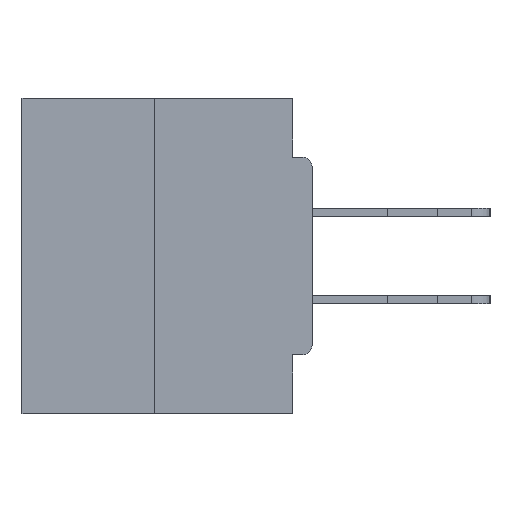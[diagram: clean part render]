
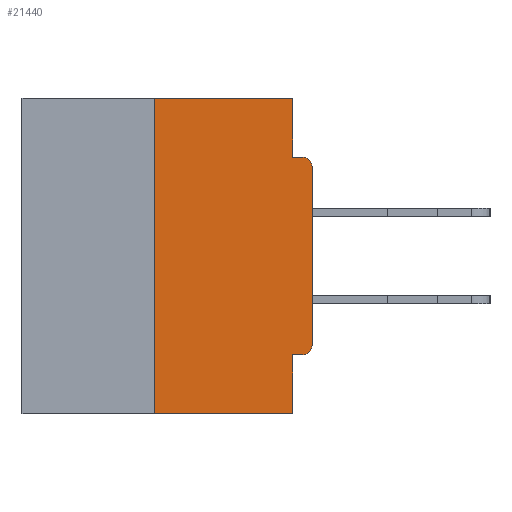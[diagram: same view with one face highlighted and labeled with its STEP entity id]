
A CAD part, left-side view. The second image highlights one B-rep face of the part: STEP entity #21440.
In plain terms, the highlighted planar face has unit normal (-1, 0, 0).
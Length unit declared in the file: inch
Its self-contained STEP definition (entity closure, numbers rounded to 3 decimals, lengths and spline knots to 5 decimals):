
#473 = VERTEX_POINT ( 'NONE', #34728 ) ;
#494 = CARTESIAN_POINT ( 'NONE',  ( 0., 0.25, 0. ) ) ;
#676 = DIRECTION ( 'NONE',  ( 0., 1., 0. ) ) ;
#697 = DIRECTION ( 'NONE',  ( 0., -1., 0. ) ) ;
#2368 = LINE ( 'NONE', #22372, #6862 ) ;
#2911 = LINE ( 'NONE', #5901, #22941 ) ;
#3877 = CARTESIAN_POINT ( 'NONE',  ( 0., 0., -0.4065 ) ) ;
#5074 = CARTESIAN_POINT ( 'NONE',  ( 0., 0.46, 0. ) ) ;
#5537 = CARTESIAN_POINT ( 'NONE',  ( 0., 0.015, -0.4065 ) ) ;
#5901 = CARTESIAN_POINT ( 'NONE',  ( 0., 0.25, 0. ) ) ;
#6268 = CIRCLE ( 'NONE', #41624, 0.015 ) ;
#6456 = VERTEX_POINT ( 'NONE', #11626 ) ;
#6700 = EDGE_CURVE ( 'NONE', #13924, #473, #20686, .T. ) ;
#6862 = VECTOR ( 'NONE', #24736, 39.37008 ) ;
#7911 = VERTEX_POINT ( 'NONE', #41515 ) ;
#8162 = VECTOR ( 'NONE', #697, 39.37008 ) ;
#8519 = CARTESIAN_POINT ( 'NONE',  ( 0., 0.031, -0.5 ) ) ;
#8876 = DIRECTION ( 'NONE',  ( -1., 0., 0. ) ) ;
#9008 = CARTESIAN_POINT ( 'NONE',  ( 0., 0.031, -0.5 ) ) ;
#9413 = ORIENTED_EDGE ( 'NONE', *, *, #31397, .F. ) ;
#9829 = LINE ( 'NONE', #17039, #32556 ) ;
#10987 = DIRECTION ( 'NONE',  ( -1., 0., 0. ) ) ;
#11491 = ORIENTED_EDGE ( 'NONE', *, *, #18072, .T. ) ;
#11492 = VERTEX_POINT ( 'NONE', #39546 ) ;
#11626 = CARTESIAN_POINT ( 'NONE',  ( 0., 0.031, 0. ) ) ;
#11719 = VECTOR ( 'NONE', #18060, 39.37008 ) ;
#12314 = VECTOR ( 'NONE', #35559, 39.37008 ) ;
#13902 = CARTESIAN_POINT ( 'NONE',  ( 0., 0., -0.1085 ) ) ;
#13924 = VERTEX_POINT ( 'NONE', #5537 ) ;
#14106 = LINE ( 'NONE', #29868, #8162 ) ;
#14515 = VERTEX_POINT ( 'NONE', #494 ) ;
#15342 = LINE ( 'NONE', #41324, #12314 ) ;
#15355 = ORIENTED_EDGE ( 'NONE', *, *, #36718, .T. ) ;
#15449 = EDGE_CURVE ( 'NONE', #14515, #6456, #34242, .T. ) ;
#15707 = VECTOR ( 'NONE', #676, 39.37008 ) ;
#16113 = CARTESIAN_POINT ( 'NONE',  ( 0., 0., -0.3915 ) ) ;
#16138 = ORIENTED_EDGE ( 'NONE', *, *, #15449, .F. ) ;
#17039 = CARTESIAN_POINT ( 'NONE',  ( 0., 0.031, 0. ) ) ;
#17478 = ORIENTED_EDGE ( 'NONE', *, *, #41004, .F. ) ;
#18060 = DIRECTION ( 'NONE',  ( 0., -1., 0. ) ) ;
#18072 = EDGE_CURVE ( 'NONE', #13924, #34018, #26867, .T. ) ;
#19456 = DIRECTION ( 'NONE',  ( 1., 0., 0. ) ) ;
#20686 = LINE ( 'NONE', #3877, #15707 ) ;
#20988 = CARTESIAN_POINT ( 'NONE',  ( 0., 0.015, -0.3915 ) ) ;
#21440 = ADVANCED_FACE ( 'NONE', ( #38626 ), #32837, .F. ) ;
#21739 = AXIS2_PLACEMENT_3D ( 'NONE', #25638, #19456, #25832 ) ;
#21856 = DIRECTION ( 'NONE',  ( 0., 0., -1. ) ) ;
#22372 = CARTESIAN_POINT ( 'NONE',  ( 0., 0.46, -0.5 ) ) ;
#22941 = VECTOR ( 'NONE', #41046, 39.37008 ) ;
#23194 = EDGE_CURVE ( 'NONE', #11492, #26535, #2368, .T. ) ;
#24131 = AXIS2_PLACEMENT_3D ( 'NONE', #20988, #10987, #40383 ) ;
#24409 = VERTEX_POINT ( 'NONE', #39922 ) ;
#24691 = ORIENTED_EDGE ( 'NONE', *, *, #23194, .T. ) ;
#24736 = DIRECTION ( 'NONE',  ( 0., -1., 0. ) ) ;
#25382 = EDGE_CURVE ( 'NONE', #41087, #7911, #6268, .T. ) ;
#25638 = CARTESIAN_POINT ( 'NONE',  ( 0., 0.46, 0. ) ) ;
#25832 = DIRECTION ( 'NONE',  ( 0., 0., -1. ) ) ;
#26535 = VERTEX_POINT ( 'NONE', #8519 ) ;
#26867 = CIRCLE ( 'NONE', #24131, 0.015 ) ;
#26870 = VECTOR ( 'NONE', #37972, 39.37008 ) ;
#28997 = ORIENTED_EDGE ( 'NONE', *, *, #29095, .F. ) ;
#29095 = EDGE_CURVE ( 'NONE', #473, #26535, #37333, .T. ) ;
#29868 = CARTESIAN_POINT ( 'NONE',  ( 0., 0., -0.0935 ) ) ;
#31397 = EDGE_CURVE ( 'NONE', #11492, #14515, #2911, .T. ) ;
#32556 = VECTOR ( 'NONE', #35810, 39.37008 ) ;
#32837 = PLANE ( 'NONE',  #21739 ) ;
#33560 = ORIENTED_EDGE ( 'NONE', *, *, #6700, .F. ) ;
#34018 = VERTEX_POINT ( 'NONE', #16113 ) ;
#34242 = LINE ( 'NONE', #5074, #11719 ) ;
#34728 = CARTESIAN_POINT ( 'NONE',  ( 0., 0.031, -0.4065 ) ) ;
#35272 = ORIENTED_EDGE ( 'NONE', *, *, #40176, .F. ) ;
#35559 = DIRECTION ( 'NONE',  ( 0., 0., 1. ) ) ;
#35810 = DIRECTION ( 'NONE',  ( 0., 0., -1. ) ) ;
#36718 = EDGE_CURVE ( 'NONE', #34018, #41087, #15342, .T. ) ;
#37333 = LINE ( 'NONE', #9008, #26870 ) ;
#37972 = DIRECTION ( 'NONE',  ( 0., 0., -1. ) ) ;
#38626 = FACE_OUTER_BOUND ( 'NONE', #39864, .T. ) ;
#38670 = ORIENTED_EDGE ( 'NONE', *, *, #25382, .T. ) ;
#39546 = CARTESIAN_POINT ( 'NONE',  ( 0., 0.25, -0.5 ) ) ;
#39864 = EDGE_LOOP ( 'NONE', ( #16138, #9413, #24691, #28997, #33560, #11491, #15355, #38670, #17478, #35272 ) ) ;
#39922 = CARTESIAN_POINT ( 'NONE',  ( 0., 0.031, -0.0935 ) ) ;
#40176 = EDGE_CURVE ( 'NONE', #6456, #24409, #9829, .T. ) ;
#40383 = DIRECTION ( 'NONE',  ( 0., 0., -1. ) ) ;
#40822 = CARTESIAN_POINT ( 'NONE',  ( 0., 0.015, -0.1085 ) ) ;
#41004 = EDGE_CURVE ( 'NONE', #24409, #7911, #14106, .T. ) ;
#41046 = DIRECTION ( 'NONE',  ( 0., 0., 1. ) ) ;
#41087 = VERTEX_POINT ( 'NONE', #13902 ) ;
#41324 = CARTESIAN_POINT ( 'NONE',  ( 0., 0., 0. ) ) ;
#41515 = CARTESIAN_POINT ( 'NONE',  ( 0., 0.015, -0.0935 ) ) ;
#41624 = AXIS2_PLACEMENT_3D ( 'NONE', #40822, #8876, #21856 ) ;
